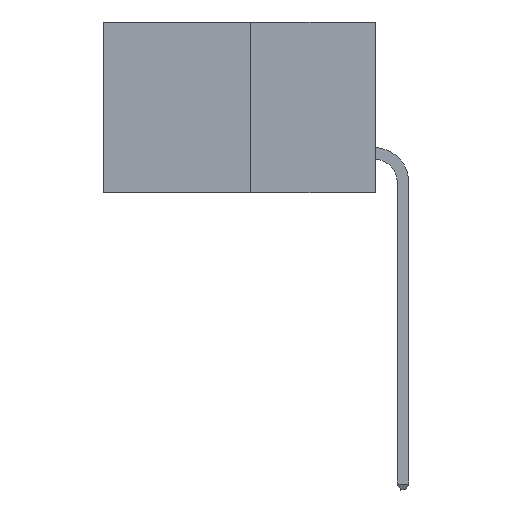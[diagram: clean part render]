
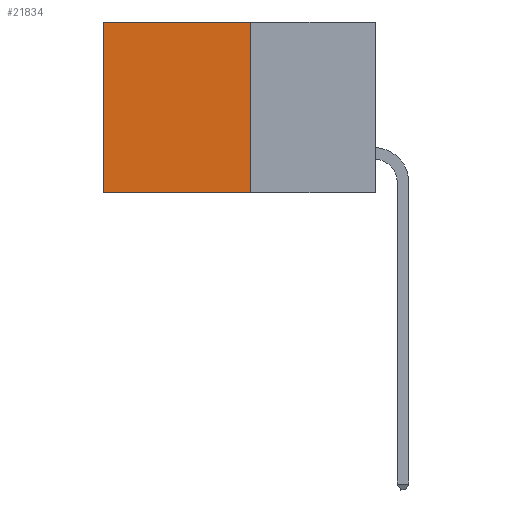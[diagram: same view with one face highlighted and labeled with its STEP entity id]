
A CAD part, left-side view. The second image highlights one B-rep face of the part: STEP entity #21834.
In plain terms, the highlighted planar face has unit normal (-1, 0, 0).
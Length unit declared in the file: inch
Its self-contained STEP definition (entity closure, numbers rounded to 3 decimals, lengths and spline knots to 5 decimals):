
#841 = CARTESIAN_POINT ( 'NONE',  ( 0.277, 0.59, 0. ) ) ;
#944 = CARTESIAN_POINT ( 'NONE',  ( 0.277, 0.27, -0.37 ) ) ;
#1090 = LINE ( 'NONE', #944, #6568 ) ;
#1796 = CARTESIAN_POINT ( 'NONE',  ( 0.277, 0.59, -0.37 ) ) ;
#2628 = VERTEX_POINT ( 'NONE', #20039 ) ;
#2651 = ORIENTED_EDGE ( 'NONE', *, *, #11376, .T. ) ;
#3672 = CARTESIAN_POINT ( 'NONE',  ( 0.277, 0.27, 0. ) ) ;
#4706 = PLANE ( 'NONE',  #20711 ) ;
#5312 = LINE ( 'NONE', #33882, #11503 ) ;
#5563 = DIRECTION ( 'NONE',  ( 0., 1., 0. ) ) ;
#5822 = VERTEX_POINT ( 'NONE', #841 ) ;
#6568 = VECTOR ( 'NONE', #16846, 39.37008 ) ;
#7380 = DIRECTION ( 'NONE',  ( 0., 0., -1. ) ) ;
#8987 = ORIENTED_EDGE ( 'NONE', *, *, #17797, .T. ) ;
#9569 = VERTEX_POINT ( 'NONE', #3672 ) ;
#9835 = DIRECTION ( 'NONE',  ( 0., 0., -1. ) ) ;
#10706 = FACE_OUTER_BOUND ( 'NONE', #28256, .T. ) ;
#11376 = EDGE_CURVE ( 'NONE', #9569, #5822, #24382, .T. ) ;
#11503 = VECTOR ( 'NONE', #26306, 39.37008 ) ;
#13773 = EDGE_CURVE ( 'NONE', #33728, #2628, #5312, .T. ) ;
#16846 = DIRECTION ( 'NONE',  ( 0., 0., -1. ) ) ;
#17797 = EDGE_CURVE ( 'NONE', #5822, #2628, #33682, .T. ) ;
#17885 = CARTESIAN_POINT ( 'NONE',  ( 0.277, 0.27, -0.37 ) ) ;
#18551 = ORIENTED_EDGE ( 'NONE', *, *, #13773, .F. ) ;
#20039 = CARTESIAN_POINT ( 'NONE',  ( 0.277, 0.59, -0.37 ) ) ;
#20711 = AXIS2_PLACEMENT_3D ( 'NONE', #17885, #23189, #7380 ) ;
#21834 = ADVANCED_FACE ( 'NONE', ( #10706 ), #4706, .F. ) ;
#22365 = EDGE_CURVE ( 'NONE', #9569, #33728, #1090, .T. ) ;
#23189 = DIRECTION ( 'NONE',  ( 1., 0., 0. ) ) ;
#24382 = LINE ( 'NONE', #31655, #25199 ) ;
#25199 = VECTOR ( 'NONE', #5563, 39.37008 ) ;
#26306 = DIRECTION ( 'NONE',  ( 0., 1., 0. ) ) ;
#26913 = VECTOR ( 'NONE', #9835, 39.37008 ) ;
#28256 = EDGE_LOOP ( 'NONE', ( #8987, #18551, #32112, #2651 ) ) ;
#29094 = CARTESIAN_POINT ( 'NONE',  ( 0.277, 0.27, -0.37 ) ) ;
#31655 = CARTESIAN_POINT ( 'NONE',  ( 0.277, 0.27, 0. ) ) ;
#32112 = ORIENTED_EDGE ( 'NONE', *, *, #22365, .F. ) ;
#33682 = LINE ( 'NONE', #1796, #26913 ) ;
#33728 = VERTEX_POINT ( 'NONE', #29094 ) ;
#33882 = CARTESIAN_POINT ( 'NONE',  ( 0.277, 0.27, -0.37 ) ) ;
